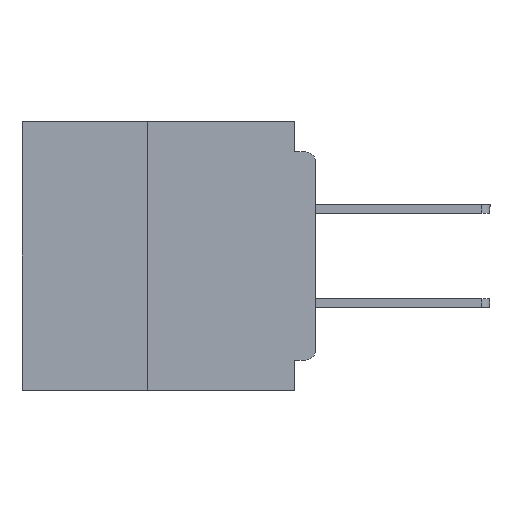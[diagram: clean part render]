
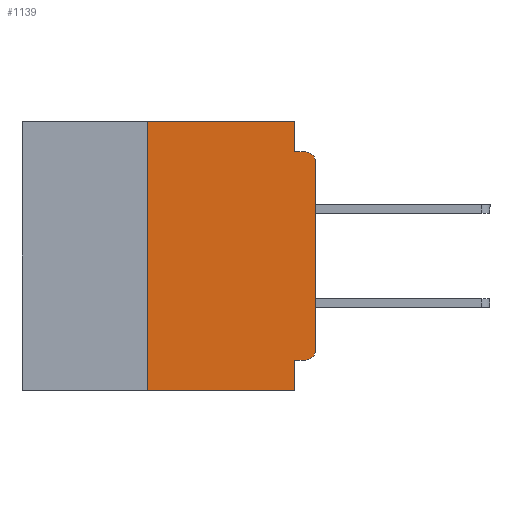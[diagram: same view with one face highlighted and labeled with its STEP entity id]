
A CAD part, left-side view. The second image highlights one B-rep face of the part: STEP entity #1139.
In plain terms, the highlighted planar face has unit normal (-1, 0, 0).
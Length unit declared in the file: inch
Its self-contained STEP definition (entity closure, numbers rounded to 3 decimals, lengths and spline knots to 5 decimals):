
#1139 = ADVANCED_FACE ( 'NONE', ( #37011 ), #8579, .F. ) ;
#2494 = VECTOR ( 'NONE', #8543, 39.37008 ) ;
#3501 = DIRECTION ( 'NONE',  ( 0., -1., 0. ) ) ;
#4066 = VECTOR ( 'NONE', #39518, 39.37008 ) ;
#4378 = DIRECTION ( 'NONE',  ( 0., 1., 0. ) ) ;
#5113 = LINE ( 'NONE', #30118, #4066 ) ;
#5818 = DIRECTION ( 'NONE',  ( 0., -1., 0. ) ) ;
#6054 = CARTESIAN_POINT ( 'NONE',  ( 0., 0.015, -0.34 ) ) ;
#6717 = CARTESIAN_POINT ( 'NONE',  ( 0., 0., -0.34 ) ) ;
#7097 = VERTEX_POINT ( 'NONE', #23201 ) ;
#7512 = CARTESIAN_POINT ( 'NONE',  ( 0., 0., -0.355 ) ) ;
#7653 = EDGE_CURVE ( 'NONE', #36743, #37027, #10705, .T. ) ;
#8214 = VERTEX_POINT ( 'NONE', #32187 ) ;
#8543 = DIRECTION ( 'NONE',  ( 0., 0., -1. ) ) ;
#8579 = PLANE ( 'NONE',  #36052 ) ;
#8685 = EDGE_CURVE ( 'NONE', #20427, #11487, #19627, .T. ) ;
#8973 = VERTEX_POINT ( 'NONE', #6717 ) ;
#9265 = DIRECTION ( 'NONE',  ( 0., 0., -1. ) ) ;
#9534 = EDGE_CURVE ( 'NONE', #37027, #20427, #14064, .T. ) ;
#10392 = CARTESIAN_POINT ( 'NONE',  ( 0., 0.015, -0.06 ) ) ;
#10705 = LINE ( 'NONE', #38609, #24778 ) ;
#11009 = CARTESIAN_POINT ( 'NONE',  ( 0., 0.031, -0.4 ) ) ;
#11355 = ORIENTED_EDGE ( 'NONE', *, *, #29780, .T. ) ;
#11487 = VERTEX_POINT ( 'NONE', #32029 ) ;
#11607 = ORIENTED_EDGE ( 'NONE', *, *, #7653, .F. ) ;
#12139 = CARTESIAN_POINT ( 'NONE',  ( 0., 0.437, 0. ) ) ;
#12298 = ORIENTED_EDGE ( 'NONE', *, *, #9534, .F. ) ;
#12460 = ORIENTED_EDGE ( 'NONE', *, *, #8685, .F. ) ;
#13224 = ORIENTED_EDGE ( 'NONE', *, *, #19217, .F. ) ;
#13603 = EDGE_CURVE ( 'NONE', #30057, #7097, #37470, .T. ) ;
#13648 = DIRECTION ( 'NONE',  ( 0., 0., -1. ) ) ;
#13829 = ORIENTED_EDGE ( 'NONE', *, *, #35792, .T. ) ;
#13915 = CIRCLE ( 'NONE', #41224, 0.015 ) ;
#14064 = LINE ( 'NONE', #32295, #37536 ) ;
#14119 = ORIENTED_EDGE ( 'NONE', *, *, #18433, .T. ) ;
#14388 = EDGE_CURVE ( 'NONE', #30057, #8973, #13915, .T. ) ;
#15516 = VECTOR ( 'NONE', #36577, 39.37008 ) ;
#18433 = EDGE_CURVE ( 'NONE', #8973, #27455, #22650, .T. ) ;
#18721 = ORIENTED_EDGE ( 'NONE', *, *, #13603, .F. ) ;
#18804 = DIRECTION ( 'NONE',  ( 1., 0., 0. ) ) ;
#18843 = DIRECTION ( 'NONE',  ( 0., 0., -1. ) ) ;
#19217 = EDGE_CURVE ( 'NONE', #11487, #8214, #34046, .T. ) ;
#19627 = LINE ( 'NONE', #27639, #2494 ) ;
#20190 = EDGE_LOOP ( 'NONE', ( #14119, #13829, #13224, #12460, #12298, #11607, #11355, #32968, #18721, #37331 ) ) ;
#20427 = VERTEX_POINT ( 'NONE', #25840 ) ;
#22650 = LINE ( 'NONE', #30576, #31192 ) ;
#22728 = DIRECTION ( 'NONE',  ( 0., 0., 1. ) ) ;
#23137 = CARTESIAN_POINT ( 'NONE',  ( 0., 0.031, -0.4 ) ) ;
#23201 = CARTESIAN_POINT ( 'NONE',  ( 0., 0.031, -0.355 ) ) ;
#24176 = CIRCLE ( 'NONE', #31382, 0.015 ) ;
#24778 = VECTOR ( 'NONE', #22728, 39.37008 ) ;
#24803 = CARTESIAN_POINT ( 'NONE',  ( 0., 0.25, -0.4 ) ) ;
#25180 = CARTESIAN_POINT ( 'NONE',  ( 0., 0.015, -0.355 ) ) ;
#25613 = VECTOR ( 'NONE', #5818, 39.37008 ) ;
#25840 = CARTESIAN_POINT ( 'NONE',  ( 0., 0.031, 0. ) ) ;
#27455 = VERTEX_POINT ( 'NONE', #37692 ) ;
#27639 = CARTESIAN_POINT ( 'NONE',  ( 0., 0.031, 0. ) ) ;
#28381 = VERTEX_POINT ( 'NONE', #23137 ) ;
#28495 = DIRECTION ( 'NONE',  ( -1., 0., 0. ) ) ;
#29780 = EDGE_CURVE ( 'NONE', #36743, #28381, #5113, .T. ) ;
#30057 = VERTEX_POINT ( 'NONE', #25180 ) ;
#30118 = CARTESIAN_POINT ( 'NONE',  ( 0., 0.437, -0.4 ) ) ;
#30576 = CARTESIAN_POINT ( 'NONE',  ( 0., 0., 0. ) ) ;
#31192 = VECTOR ( 'NONE', #40108, 39.37008 ) ;
#31382 = AXIS2_PLACEMENT_3D ( 'NONE', #10392, #32807, #13648 ) ;
#32029 = CARTESIAN_POINT ( 'NONE',  ( 0., 0.031, -0.045 ) ) ;
#32187 = CARTESIAN_POINT ( 'NONE',  ( 0., 0.015, -0.045 ) ) ;
#32295 = CARTESIAN_POINT ( 'NONE',  ( 0., 0.437, 0. ) ) ;
#32541 = LINE ( 'NONE', #11009, #15516 ) ;
#32807 = DIRECTION ( 'NONE',  ( -1., 0., 0. ) ) ;
#32968 = ORIENTED_EDGE ( 'NONE', *, *, #37075, .F. ) ;
#34046 = LINE ( 'NONE', #37560, #25613 ) ;
#35792 = EDGE_CURVE ( 'NONE', #27455, #8214, #24176, .T. ) ;
#36052 = AXIS2_PLACEMENT_3D ( 'NONE', #12139, #18804, #18843 ) ;
#36472 = VECTOR ( 'NONE', #4378, 39.37008 ) ;
#36577 = DIRECTION ( 'NONE',  ( 0., 0., -1. ) ) ;
#36743 = VERTEX_POINT ( 'NONE', #24803 ) ;
#37011 = FACE_OUTER_BOUND ( 'NONE', #20190, .T. ) ;
#37027 = VERTEX_POINT ( 'NONE', #39509 ) ;
#37075 = EDGE_CURVE ( 'NONE', #7097, #28381, #32541, .T. ) ;
#37331 = ORIENTED_EDGE ( 'NONE', *, *, #14388, .T. ) ;
#37470 = LINE ( 'NONE', #7512, #36472 ) ;
#37536 = VECTOR ( 'NONE', #3501, 39.37008 ) ;
#37560 = CARTESIAN_POINT ( 'NONE',  ( 0., 0., -0.045 ) ) ;
#37692 = CARTESIAN_POINT ( 'NONE',  ( 0., 0., -0.06 ) ) ;
#38609 = CARTESIAN_POINT ( 'NONE',  ( 0., 0.25, -0.4 ) ) ;
#39509 = CARTESIAN_POINT ( 'NONE',  ( 0., 0.25, 0. ) ) ;
#39518 = DIRECTION ( 'NONE',  ( 0., -1., 0. ) ) ;
#40108 = DIRECTION ( 'NONE',  ( 0., 0., 1. ) ) ;
#41224 = AXIS2_PLACEMENT_3D ( 'NONE', #6054, #28495, #9265 ) ;
